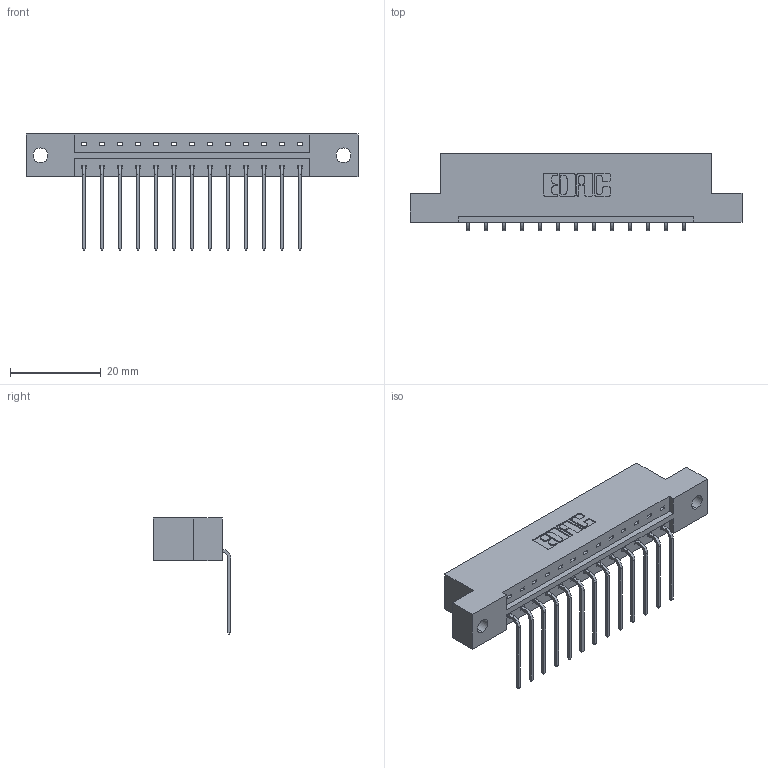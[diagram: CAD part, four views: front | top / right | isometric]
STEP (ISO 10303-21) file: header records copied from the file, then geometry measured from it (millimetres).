
FILE_DESCRIPTION (( 'STEP AP203' ), '1' );
FILE_NAME ('833-013-559-102.STEP', '2020-05-31T00:34:25', ( '' ), ( '' ), 'SwSTEP 2.0', 'SolidWorks 2020', '' );
FILE_SCHEMA (( 'CONFIG_CONTROL_DESIGN' ));
Length unit declared in the file: inch
Products named in the file (3): 833-013-559-102; 833 Part_Flush - .128 Dia; 345-292-001_558 559 Tail - 1
Assembly tree (14 placements, depth 2):
  833-013-559-102
    833 Part_Flush - .128 Dia
    345-292-001_558 559 Tail - 1  x13
Bounding box: 73.05 x 17.09 x 25.53 mm (x, y, z)
Volume: 7108.2 mm3; surface area: 7494.4 mm2
Topology: 14 solids, 14 shells, 894 faces, 2677 edges, 1766 vertices
Faces by surface type: plane 642, cylinder 252
Entity records: 11785 total; most frequent: CARTESIAN_POINT 2045, ORIENTED_EDGE 1994, DIRECTION 1783, EDGE_CURVE 997, LINE 869, VECTOR 869, VERTEX_POINT 662, AXIS2_PLACEMENT_3D 457
